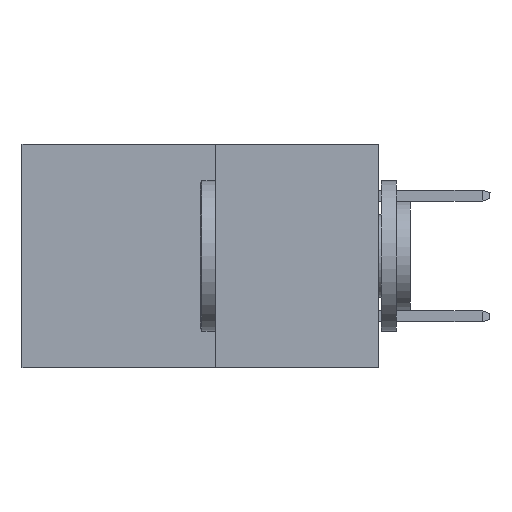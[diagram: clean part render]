
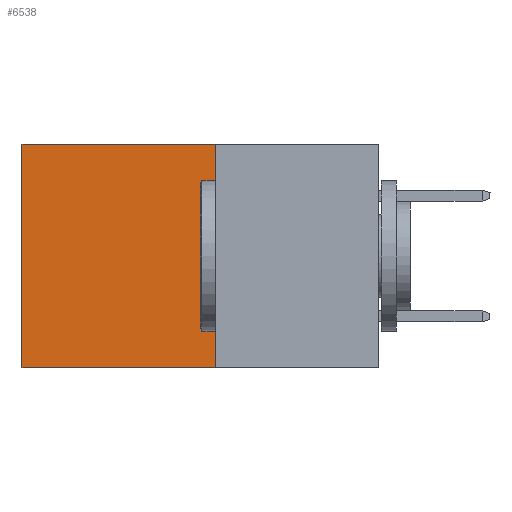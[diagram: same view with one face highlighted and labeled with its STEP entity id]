
A CAD part, left-side view. The second image highlights one B-rep face of the part: STEP entity #6538.
In plain terms, the highlighted planar face has unit normal (-1, 0, 0).
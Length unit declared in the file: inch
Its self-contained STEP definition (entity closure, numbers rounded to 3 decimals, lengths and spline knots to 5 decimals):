
#1026 = LINE ( 'NONE', #9058, #3326 ) ;
#1214 = ORIENTED_EDGE ( 'NONE', *, *, #6815, .F. ) ;
#1942 = CARTESIAN_POINT ( 'NONE',  ( 0.277, 0.59, -0.37 ) ) ;
#2014 = PLANE ( 'NONE',  #10510 ) ;
#2165 = EDGE_CURVE ( 'NONE', #9658, #7659, #6523, .T. ) ;
#2444 = LINE ( 'NONE', #11367, #9309 ) ;
#2546 = DIRECTION ( 'NONE',  ( 0., 1., 0. ) ) ;
#2674 = CARTESIAN_POINT ( 'NONE',  ( 0.277, 0.59, 0. ) ) ;
#2894 = FACE_OUTER_BOUND ( 'NONE', #3213, .T. ) ;
#3213 = EDGE_LOOP ( 'NONE', ( #8523, #10933, #1214, #6459 ) ) ;
#3326 = VECTOR ( 'NONE', #2546, 39.37008 ) ;
#3346 = VERTEX_POINT ( 'NONE', #8476 ) ;
#4986 = CARTESIAN_POINT ( 'NONE',  ( 0.277, 0.27, -0.37 ) ) ;
#5980 = DIRECTION ( 'NONE',  ( 0., 1., 0. ) ) ;
#6271 = CARTESIAN_POINT ( 'NONE',  ( 0.277, 0.59, -0.37 ) ) ;
#6459 = ORIENTED_EDGE ( 'NONE', *, *, #2165, .T. ) ;
#6523 = LINE ( 'NONE', #8355, #11277 ) ;
#6538 = ADVANCED_FACE ( 'NONE', ( #2894 ), #2014, .F. ) ;
#6660 = DIRECTION ( 'NONE',  ( 0., 0., -1. ) ) ;
#6815 = EDGE_CURVE ( 'NONE', #9658, #3346, #2444, .T. ) ;
#7567 = EDGE_CURVE ( 'NONE', #3346, #9692, #1026, .T. ) ;
#7659 = VERTEX_POINT ( 'NONE', #2674 ) ;
#8355 = CARTESIAN_POINT ( 'NONE',  ( 0.277, 0.27, 0. ) ) ;
#8476 = CARTESIAN_POINT ( 'NONE',  ( 0.277, 0.27, -0.37 ) ) ;
#8523 = ORIENTED_EDGE ( 'NONE', *, *, #11901, .T. ) ;
#9058 = CARTESIAN_POINT ( 'NONE',  ( 0.277, 0.27, -0.37 ) ) ;
#9201 = VECTOR ( 'NONE', #11630, 39.37008 ) ;
#9309 = VECTOR ( 'NONE', #6660, 39.37008 ) ;
#9399 = CARTESIAN_POINT ( 'NONE',  ( 0.277, 0.27, 0. ) ) ;
#9473 = LINE ( 'NONE', #6271, #9201 ) ;
#9658 = VERTEX_POINT ( 'NONE', #9399 ) ;
#9692 = VERTEX_POINT ( 'NONE', #1942 ) ;
#10262 = DIRECTION ( 'NONE',  ( 1., 0., 0. ) ) ;
#10410 = DIRECTION ( 'NONE',  ( 0., 0., -1. ) ) ;
#10510 = AXIS2_PLACEMENT_3D ( 'NONE', #4986, #10262, #10410 ) ;
#10933 = ORIENTED_EDGE ( 'NONE', *, *, #7567, .F. ) ;
#11277 = VECTOR ( 'NONE', #5980, 39.37008 ) ;
#11367 = CARTESIAN_POINT ( 'NONE',  ( 0.277, 0.27, -0.37 ) ) ;
#11630 = DIRECTION ( 'NONE',  ( 0., 0., -1. ) ) ;
#11901 = EDGE_CURVE ( 'NONE', #7659, #9692, #9473, .T. ) ;
